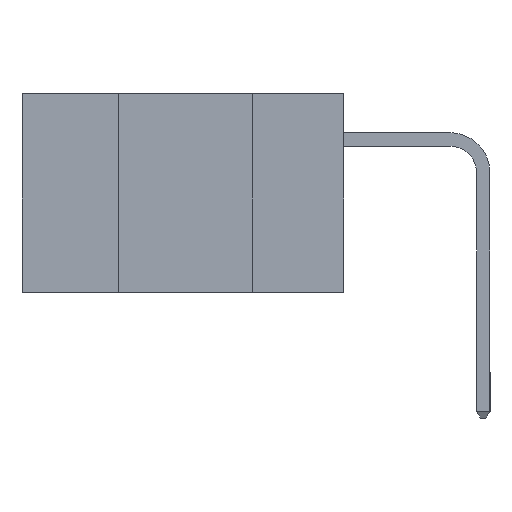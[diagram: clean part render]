
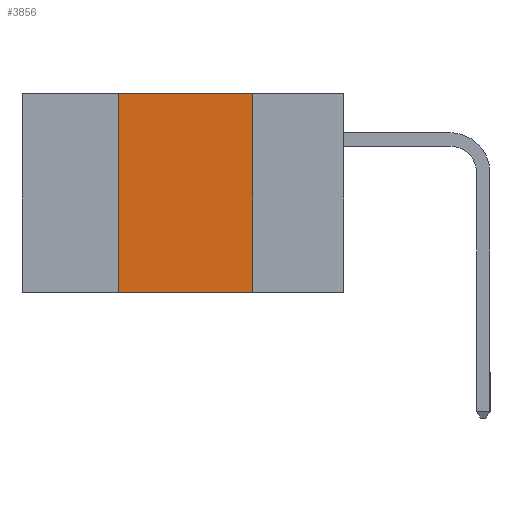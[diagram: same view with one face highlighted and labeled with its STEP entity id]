
A CAD part, left-side view. The second image highlights one B-rep face of the part: STEP entity #3856.
In plain terms, the highlighted planar face has unit normal (-1, 0, 0).
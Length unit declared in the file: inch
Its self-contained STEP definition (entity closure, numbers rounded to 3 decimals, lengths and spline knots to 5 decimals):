
#266 = DIRECTION ( 'NONE',  ( 0., 0., 1. ) ) ;
#1000 = VERTEX_POINT ( 'NONE', #21953 ) ;
#3193 = AXIS2_PLACEMENT_3D ( 'NONE', #14135, #22987, #10482 ) ;
#3856 = ADVANCED_FACE ( 'NONE', ( #16385 ), #9952, .F. ) ;
#7278 = ORIENTED_EDGE ( 'NONE', *, *, #20236, .F. ) ;
#7702 = VECTOR ( 'NONE', #8319, 39.37008 ) ;
#7848 = LINE ( 'NONE', #23193, #21879 ) ;
#7966 = VECTOR ( 'NONE', #24996, 39.37008 ) ;
#8319 = DIRECTION ( 'NONE',  ( 0., 0., -1. ) ) ;
#9952 = PLANE ( 'NONE',  #3193 ) ;
#10181 = EDGE_CURVE ( 'NONE', #25923, #1000, #26253, .T. ) ;
#10294 = CARTESIAN_POINT ( 'NONE',  ( 0., 0.42, 0. ) ) ;
#10482 = DIRECTION ( 'NONE',  ( 0., 0., -1. ) ) ;
#13866 = LINE ( 'NONE', #25785, #26935 ) ;
#14135 = CARTESIAN_POINT ( 'NONE',  ( 0., 0.6, 0. ) ) ;
#14489 = CARTESIAN_POINT ( 'NONE',  ( 0., 0.6, -0.37 ) ) ;
#16187 = CARTESIAN_POINT ( 'NONE',  ( 0., 0.42, -0.37 ) ) ;
#16385 = FACE_OUTER_BOUND ( 'NONE', #18479, .T. ) ;
#16487 = LINE ( 'NONE', #18504, #7702 ) ;
#16532 = ORIENTED_EDGE ( 'NONE', *, *, #19976, .F. ) ;
#16782 = VERTEX_POINT ( 'NONE', #10294 ) ;
#17507 = EDGE_CURVE ( 'NONE', #25923, #16782, #7848, .T. ) ;
#17998 = CARTESIAN_POINT ( 'NONE',  ( 0., 0.17, 0. ) ) ;
#18479 = EDGE_LOOP ( 'NONE', ( #16532, #7278, #25107, #21727 ) ) ;
#18504 = CARTESIAN_POINT ( 'NONE',  ( 0., 0.17, 0. ) ) ;
#19227 = VERTEX_POINT ( 'NONE', #17998 ) ;
#19976 = EDGE_CURVE ( 'NONE', #19227, #1000, #16487, .T. ) ;
#20236 = EDGE_CURVE ( 'NONE', #16782, #19227, #13866, .T. ) ;
#21727 = ORIENTED_EDGE ( 'NONE', *, *, #10181, .T. ) ;
#21879 = VECTOR ( 'NONE', #266, 39.37008 ) ;
#21953 = CARTESIAN_POINT ( 'NONE',  ( 0., 0.17, -0.37 ) ) ;
#22987 = DIRECTION ( 'NONE',  ( 1., 0., 0. ) ) ;
#23193 = CARTESIAN_POINT ( 'NONE',  ( 0., 0.42, 0. ) ) ;
#24996 = DIRECTION ( 'NONE',  ( 0., -1., 0. ) ) ;
#25107 = ORIENTED_EDGE ( 'NONE', *, *, #17507, .F. ) ;
#25785 = CARTESIAN_POINT ( 'NONE',  ( 0., 0.6, 0. ) ) ;
#25923 = VERTEX_POINT ( 'NONE', #16187 ) ;
#26054 = DIRECTION ( 'NONE',  ( 0., -1., 0. ) ) ;
#26253 = LINE ( 'NONE', #14489, #7966 ) ;
#26935 = VECTOR ( 'NONE', #26054, 39.37008 ) ;
